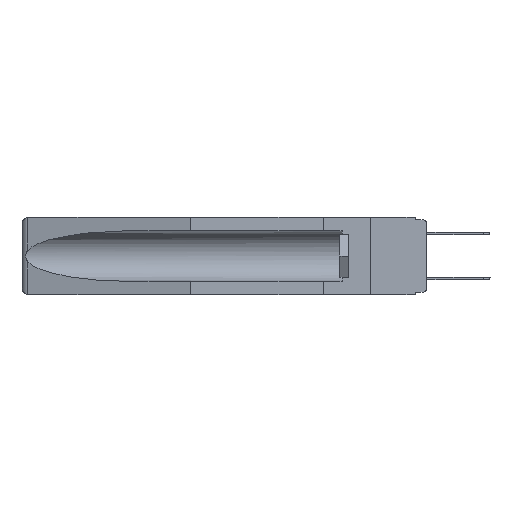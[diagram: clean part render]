
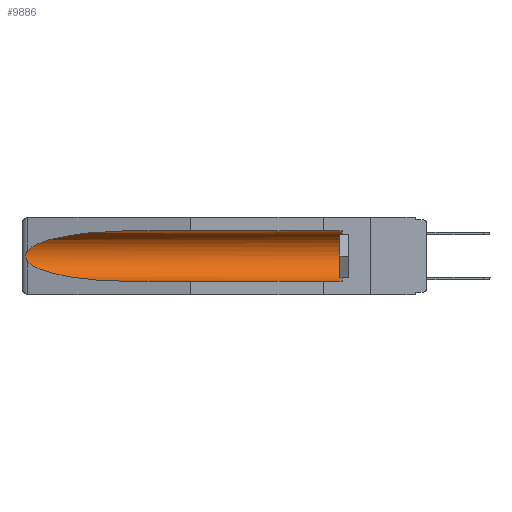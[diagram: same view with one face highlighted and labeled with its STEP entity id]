
A CAD part, left-side view. The second image highlights one B-rep face of the part: STEP entity #9886.
In plain terms, the highlighted cylindrical face has radius 2.857 mm (diameter 5.715 mm), a partial arc.
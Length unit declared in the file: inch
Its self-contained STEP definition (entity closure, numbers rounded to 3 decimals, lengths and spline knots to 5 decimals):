
#81 = DIRECTION ( 'NONE',  ( 0., 1., 0. ) ) ;
#451 = CARTESIAN_POINT ( 'NONE',  ( 0.26537, 1.52718, -0.19328 ) ) ;
#1438 = B_SPLINE_CURVE_WITH_KNOTS ( 'NONE', 3,
 ( #6692, #19489, #3022, #8548, #10545, #14217, #12134, #17814, #14133, #15904 ),
 .UNSPECIFIED., .F., .F.,
 ( 4, 2, 2, 2, 4 ),
 ( 0., 0.00029, 0.00058, 0.00087, 0.00117 ),
 .UNSPECIFIED. ) ;
#1506 = AXIS2_PLACEMENT_3D ( 'NONE', #12899, #21889, #11131 ) ;
#1562 = DIRECTION ( 'NONE',  ( 0., 1., 0. ) ) ;
#1590 = CYLINDRICAL_SURFACE ( 'NONE', #6200, 0.1125 ) ;
#3022 = CARTESIAN_POINT ( 'NONE',  ( 0.26654, 1.53092, -0.15636 ) ) ;
#3646 = VERTEX_POINT ( 'NONE', #18903 ) ;
#3774 = CARTESIAN_POINT ( 'NONE',  ( 0.155, 0.126, -0.284 ) ) ;
#4292 = EDGE_CURVE ( 'NONE', #17426, #3646, #11713, .T. ) ;
#4503 = ORIENTED_EDGE ( 'NONE', *, *, #14935, .F. ) ;
#4689 = VERTEX_POINT ( 'NONE', #7894 ) ;
#5823 = VECTOR ( 'NONE', #1562, 39.37008 ) ;
#5935 = CARTESIAN_POINT ( 'NONE',  ( 0.155, 1.07973, -0.284 ) ) ;
#6099 = ORIENTED_EDGE ( 'NONE', *, *, #11333, .T. ) ;
#6200 = AXIS2_PLACEMENT_3D ( 'NONE', #8050, #20835, #11736 ) ;
#6213 = CARTESIAN_POINT ( 'NONE',  ( 0.26537, 1.52718, -0.19328 ) ) ;
#6692 = CARTESIAN_POINT ( 'NONE',  ( 0.26537, 1.52718, -0.14972 ) ) ;
#6897 = CARTESIAN_POINT ( 'NONE',  ( 0.21114, 1.30732, -0.059 ) ) ;
#7468 = VERTEX_POINT ( 'NONE', #21678 ) ;
#7551 = ORIENTED_EDGE ( 'NONE', *, *, #7631, .T. ) ;
#7631 = EDGE_CURVE ( 'NONE', #23705, #17426, #1438, .T. ) ;
#7894 = CARTESIAN_POINT ( 'NONE',  ( 0.155, 0.126, -0.059 ) ) ;
#8050 = CARTESIAN_POINT ( 'NONE',  ( 0.155, -0.30754, -0.1715 ) ) ;
#8548 = CARTESIAN_POINT ( 'NONE',  ( 0.2673, 1.5327, -0.16383 ) ) ;
#9320 = ORIENTED_EDGE ( 'NONE', *, *, #17659, .T. ) ;
#9886 = ADVANCED_FACE ( 'NONE', ( #15614 ), #1590, .F. ) ;
#10159 = CARTESIAN_POINT ( 'NONE',  ( 0.21114, 1.30732, -0.284 ) ) ;
#10545 = CARTESIAN_POINT ( 'NONE',  ( 0.2675, 1.53308, -0.16763 ) ) ;
#10992 = CIRCLE ( 'NONE', #1506, 0.1125 ) ;
#11131 = DIRECTION ( 'NONE',  ( 0., 0., 1. ) ) ;
#11228 = CARTESIAN_POINT ( 'NONE',  ( 0.155, -0.30754, -0.284 ) ) ;
#11333 = EDGE_CURVE ( 'NONE', #4689, #7468, #21520, .T. ) ;
#11713 =( BOUNDED_CURVE ( )  B_SPLINE_CURVE ( 3, ( #451, #20698, #10159, #5935 ),
 .UNSPECIFIED., .F., .F. ) 
 B_SPLINE_CURVE_WITH_KNOTS ( ( 4, 4 ),
 ( 0.1948, 1.5708 ),
 .UNSPECIFIED. ) 
 CURVE ( )  GEOMETRIC_REPRESENTATION_ITEM ( )  RATIONAL_B_SPLINE_CURVE ( ( 1., 0.848, 0.848, 1. ) ) 
 REPRESENTATION_ITEM ( '' )  );
#11736 = DIRECTION ( 'NONE',  ( 0., 0., 1. ) ) ;
#12112 = CARTESIAN_POINT ( 'NONE',  ( 0.26537, 1.52718, -0.14972 ) ) ;
#12134 = CARTESIAN_POINT ( 'NONE',  ( 0.2673, 1.53269, -0.17917 ) ) ;
#12548 = LINE ( 'NONE', #11228, #21957 ) ;
#12899 = CARTESIAN_POINT ( 'NONE',  ( 0.155, 0.126, -0.1715 ) ) ;
#14133 = CARTESIAN_POINT ( 'NONE',  ( 0.26597, 1.5296, -0.19026 ) ) ;
#14217 = CARTESIAN_POINT ( 'NONE',  ( 0.2675, 1.53308, -0.17534 ) ) ;
#14531 = EDGE_LOOP ( 'NONE', ( #9320, #7551, #22100, #4503, #23227, #6099 ) ) ;
#14935 = EDGE_CURVE ( 'NONE', #21341, #3646, #12548, .T. ) ;
#15614 = FACE_OUTER_BOUND ( 'NONE', #14531, .T. ) ;
#15904 = CARTESIAN_POINT ( 'NONE',  ( 0.26537, 1.52718, -0.19328 ) ) ;
#16134 = CARTESIAN_POINT ( 'NONE',  ( 0.155, -0.30754, -0.059 ) ) ;
#17426 = VERTEX_POINT ( 'NONE', #6213 ) ;
#17604 = CARTESIAN_POINT ( 'NONE',  ( 0.25451, 1.48313, -0.09465 ) ) ;
#17659 = EDGE_CURVE ( 'NONE', #7468, #23705, #19607, .T. ) ;
#17684 = CARTESIAN_POINT ( 'NONE',  ( 0.155, 1.07973, -0.059 ) ) ;
#17814 = CARTESIAN_POINT ( 'NONE',  ( 0.26655, 1.53094, -0.18657 ) ) ;
#17884 = EDGE_CURVE ( 'NONE', #21341, #4689, #10992, .T. ) ;
#18903 = CARTESIAN_POINT ( 'NONE',  ( 0.155, 1.07973, -0.284 ) ) ;
#19489 = CARTESIAN_POINT ( 'NONE',  ( 0.26597, 1.52961, -0.15275 ) ) ;
#19607 =( BOUNDED_CURVE ( )  B_SPLINE_CURVE ( 3, ( #17684, #6897, #17604, #23103 ),
 .UNSPECIFIED., .F., .F. ) 
 B_SPLINE_CURVE_WITH_KNOTS ( ( 4, 4 ),
 ( 4.71239, 6.08839 ),
 .UNSPECIFIED. ) 
 CURVE ( )  GEOMETRIC_REPRESENTATION_ITEM ( )  RATIONAL_B_SPLINE_CURVE ( ( 1., 0.848, 0.848, 1. ) ) 
 REPRESENTATION_ITEM ( '' )  );
#20698 = CARTESIAN_POINT ( 'NONE',  ( 0.25451, 1.48313, -0.24835 ) ) ;
#20835 = DIRECTION ( 'NONE',  ( 0., 1., 0. ) ) ;
#21341 = VERTEX_POINT ( 'NONE', #3774 ) ;
#21520 = LINE ( 'NONE', #16134, #5823 ) ;
#21678 = CARTESIAN_POINT ( 'NONE',  ( 0.155, 1.07973, -0.059 ) ) ;
#21889 = DIRECTION ( 'NONE',  ( 0., -1., 0. ) ) ;
#21957 = VECTOR ( 'NONE', #81, 39.37008 ) ;
#22100 = ORIENTED_EDGE ( 'NONE', *, *, #4292, .T. ) ;
#23103 = CARTESIAN_POINT ( 'NONE',  ( 0.26537, 1.52718, -0.14972 ) ) ;
#23227 = ORIENTED_EDGE ( 'NONE', *, *, #17884, .T. ) ;
#23705 = VERTEX_POINT ( 'NONE', #12112 ) ;
